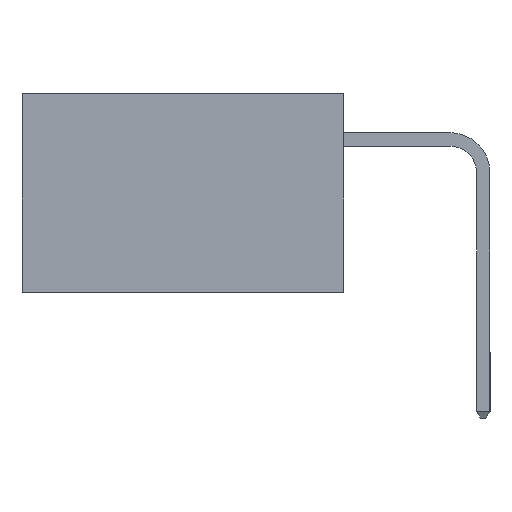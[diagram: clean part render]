
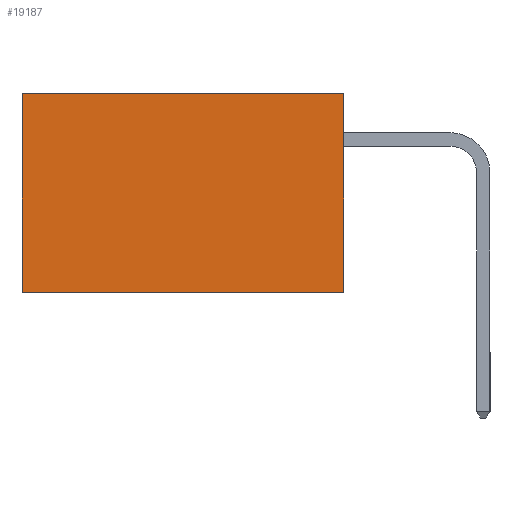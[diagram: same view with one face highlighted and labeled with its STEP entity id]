
A CAD part, left-side view. The second image highlights one B-rep face of the part: STEP entity #19187.
In plain terms, the highlighted planar face has unit normal (-1, 0, 0).
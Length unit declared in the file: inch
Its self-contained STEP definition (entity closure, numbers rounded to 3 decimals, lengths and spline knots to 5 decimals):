
#160 = VERTEX_POINT ( 'NONE', #8658 ) ;
#1061 = DIRECTION ( 'NONE',  ( 0., 0., -1. ) ) ;
#2515 = ORIENTED_EDGE ( 'NONE', *, *, #17774, .F. ) ;
#2921 = LINE ( 'NONE', #9133, #15731 ) ;
#3827 = LINE ( 'NONE', #9937, #21528 ) ;
#3834 = CARTESIAN_POINT ( 'NONE',  ( 0.298, 0.6, 0. ) ) ;
#4875 = EDGE_LOOP ( 'NONE', ( #7745, #2515, #5085, #14257 ) ) ;
#5032 = EDGE_CURVE ( 'NONE', #160, #20236, #15703, .T. ) ;
#5085 = ORIENTED_EDGE ( 'NONE', *, *, #15952, .F. ) ;
#5246 = EDGE_CURVE ( 'NONE', #20236, #22244, #2921, .T. ) ;
#5860 = CARTESIAN_POINT ( 'NONE',  ( 0.298, 0., -0.37 ) ) ;
#6243 = DIRECTION ( 'NONE',  ( 0., 0., -1. ) ) ;
#6550 = VECTOR ( 'NONE', #17761, 39.37008 ) ;
#7745 = ORIENTED_EDGE ( 'NONE', *, *, #5246, .T. ) ;
#8167 = LINE ( 'NONE', #5860, #17226 ) ;
#8658 = CARTESIAN_POINT ( 'NONE',  ( 0.298, 0., 0. ) ) ;
#9133 = CARTESIAN_POINT ( 'NONE',  ( 0.298, 0.6, 0. ) ) ;
#9698 = CARTESIAN_POINT ( 'NONE',  ( 0.298, 0., 0. ) ) ;
#9778 = FACE_OUTER_BOUND ( 'NONE', #4875, .T. ) ;
#9937 = CARTESIAN_POINT ( 'NONE',  ( 0.298, 0., 0. ) ) ;
#12336 = VERTEX_POINT ( 'NONE', #15041 ) ;
#12770 = DIRECTION ( 'NONE',  ( 0., 1., 0. ) ) ;
#13143 = PLANE ( 'NONE',  #17240 ) ;
#14257 = ORIENTED_EDGE ( 'NONE', *, *, #5032, .T. ) ;
#15041 = CARTESIAN_POINT ( 'NONE',  ( 0.298, 0., -0.37 ) ) ;
#15603 = CARTESIAN_POINT ( 'NONE',  ( 0.298, 0., 0. ) ) ;
#15703 = LINE ( 'NONE', #15603, #6550 ) ;
#15731 = VECTOR ( 'NONE', #18032, 39.37008 ) ;
#15952 = EDGE_CURVE ( 'NONE', #160, #12336, #3827, .T. ) ;
#16503 = DIRECTION ( 'NONE',  ( 1., 0., 0. ) ) ;
#17002 = CARTESIAN_POINT ( 'NONE',  ( 0.298, 0.6, -0.37 ) ) ;
#17226 = VECTOR ( 'NONE', #12770, 39.37008 ) ;
#17240 = AXIS2_PLACEMENT_3D ( 'NONE', #9698, #16503, #6243 ) ;
#17761 = DIRECTION ( 'NONE',  ( 0., 1., 0. ) ) ;
#17774 = EDGE_CURVE ( 'NONE', #12336, #22244, #8167, .T. ) ;
#18032 = DIRECTION ( 'NONE',  ( 0., 0., -1. ) ) ;
#19187 = ADVANCED_FACE ( 'NONE', ( #9778 ), #13143, .F. ) ;
#20236 = VERTEX_POINT ( 'NONE', #3834 ) ;
#21528 = VECTOR ( 'NONE', #1061, 39.37008 ) ;
#22244 = VERTEX_POINT ( 'NONE', #17002 ) ;
